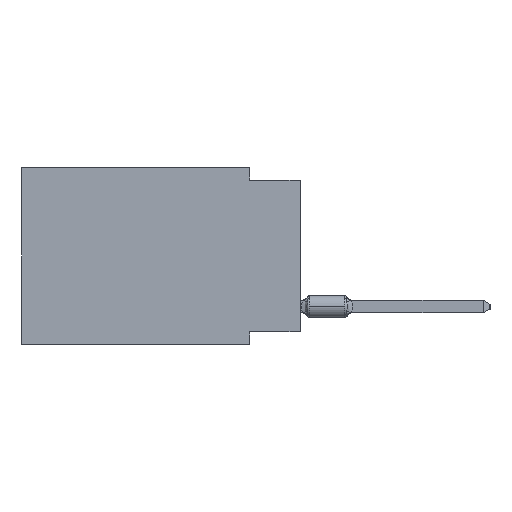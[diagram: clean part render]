
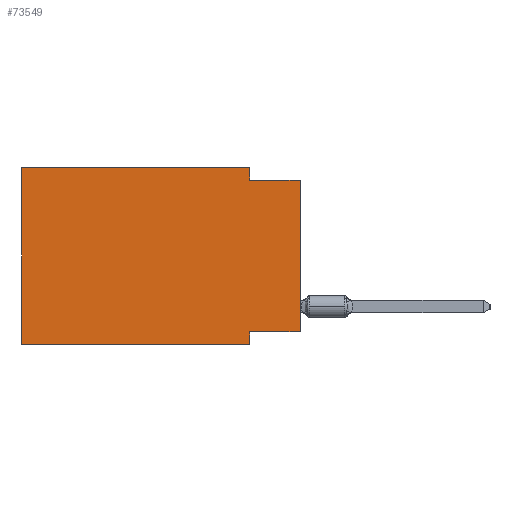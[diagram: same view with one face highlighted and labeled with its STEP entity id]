
A CAD part, left-side view. The second image highlights one B-rep face of the part: STEP entity #73549.
In plain terms, the highlighted planar face has unit normal (-1, 0, 0).
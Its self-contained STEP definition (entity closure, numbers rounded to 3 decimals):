
#684 = VERTEX_POINT ( 'NONE', #69569 ) ;
#3861 = LINE ( 'NONE', #26258, #43445 ) ;
#5385 = CARTESIAN_POINT ( 'NONE',  ( 0., 2.54, -8.89 ) ) ;
#7971 = CARTESIAN_POINT ( 'NONE',  ( 0., 0., -0.635 ) ) ;
#9413 = ORIENTED_EDGE ( 'NONE', *, *, #15101, .T. ) ;
#12250 = ORIENTED_EDGE ( 'NONE', *, *, #73054, .F. ) ;
#12953 = CARTESIAN_POINT ( 'NONE',  ( 0., 2.54, -8.255 ) ) ;
#13824 = VECTOR ( 'NONE', #46925, 1000. ) ;
#14258 = VECTOR ( 'NONE', #72425, 1000. ) ;
#15101 = EDGE_CURVE ( 'NONE', #84694, #73903, #57664, .T. ) ;
#19069 = ORIENTED_EDGE ( 'NONE', *, *, #36887, .F. ) ;
#21084 = LINE ( 'NONE', #55580, #50483 ) ;
#23249 = LINE ( 'NONE', #50221, #69173 ) ;
#25479 = ORIENTED_EDGE ( 'NONE', *, *, #57458, .F. ) ;
#26258 = CARTESIAN_POINT ( 'NONE',  ( 0., 0., 0. ) ) ;
#26704 = ORIENTED_EDGE ( 'NONE', *, *, #41740, .F. ) ;
#27658 = EDGE_CURVE ( 'NONE', #56203, #79455, #86277, .T. ) ;
#30993 = CARTESIAN_POINT ( 'NONE',  ( 0., 2.54, -8.89 ) ) ;
#31537 = FACE_OUTER_BOUND ( 'NONE', #66241, .T. ) ;
#31727 = LINE ( 'NONE', #43693, #14258 ) ;
#32801 = CARTESIAN_POINT ( 'NONE',  ( 0., 2.54, 0. ) ) ;
#36490 = VECTOR ( 'NONE', #80050, 1000. ) ;
#36887 = EDGE_CURVE ( 'NONE', #64367, #86631, #31727, .T. ) ;
#39277 = VECTOR ( 'NONE', #86770, 1000. ) ;
#41740 = EDGE_CURVE ( 'NONE', #684, #67649, #53551, .T. ) ;
#41781 = EDGE_CURVE ( 'NONE', #67649, #73903, #52700, .T. ) ;
#43445 = VECTOR ( 'NONE', #64884, 1000. ) ;
#43693 = CARTESIAN_POINT ( 'NONE',  ( 0., 0., -0.635 ) ) ;
#43954 = CARTESIAN_POINT ( 'NONE',  ( 0., 2.54, -0.635 ) ) ;
#46405 = CARTESIAN_POINT ( 'NONE',  ( 0., 13.97, -8.89 ) ) ;
#46925 = DIRECTION ( 'NONE',  ( 0., 0., -1. ) ) ;
#50221 = CARTESIAN_POINT ( 'NONE',  ( 0., 2.54, 0. ) ) ;
#50483 = VECTOR ( 'NONE', #68862, 1000. ) ;
#52297 = AXIS2_PLACEMENT_3D ( 'NONE', #52738, #79736, #72233 ) ;
#52700 = LINE ( 'NONE', #5385, #13824 ) ;
#52738 = CARTESIAN_POINT ( 'NONE',  ( 0., 13.97, 0. ) ) ;
#53551 = LINE ( 'NONE', #60193, #39277 ) ;
#55580 = CARTESIAN_POINT ( 'NONE',  ( 0., 13.97, 0. ) ) ;
#56203 = VERTEX_POINT ( 'NONE', #60008 ) ;
#56802 = DIRECTION ( 'NONE',  ( 0., -1., 0. ) ) ;
#57228 = CARTESIAN_POINT ( 'NONE',  ( 0., 13.97, -8.89 ) ) ;
#57458 = EDGE_CURVE ( 'NONE', #84694, #56203, #21084, .T. ) ;
#57664 = LINE ( 'NONE', #57228, #66122 ) ;
#59906 = DIRECTION ( 'NONE',  ( 0., 0., -1. ) ) ;
#60008 = CARTESIAN_POINT ( 'NONE',  ( 0., 13.97, 0. ) ) ;
#60193 = CARTESIAN_POINT ( 'NONE',  ( 0., 0., -8.255 ) ) ;
#64367 = VERTEX_POINT ( 'NONE', #43954 ) ;
#64884 = DIRECTION ( 'NONE',  ( 0., 0., 1. ) ) ;
#66122 = VECTOR ( 'NONE', #56802, 1000. ) ;
#66241 = EDGE_LOOP ( 'NONE', ( #79836, #19069, #12250, #69041, #25479, #9413, #79069, #26704 ) ) ;
#66777 = CARTESIAN_POINT ( 'NONE',  ( 0., 13.97, 0. ) ) ;
#67649 = VERTEX_POINT ( 'NONE', #12953 ) ;
#68862 = DIRECTION ( 'NONE',  ( 0., 0., 1. ) ) ;
#69041 = ORIENTED_EDGE ( 'NONE', *, *, #27658, .F. ) ;
#69173 = VECTOR ( 'NONE', #59906, 1000. ) ;
#69569 = CARTESIAN_POINT ( 'NONE',  ( 0., 0., -8.255 ) ) ;
#71784 = PLANE ( 'NONE',  #52297 ) ;
#72233 = DIRECTION ( 'NONE',  ( 0., 0., -1. ) ) ;
#72425 = DIRECTION ( 'NONE',  ( 0., -1., 0. ) ) ;
#73054 = EDGE_CURVE ( 'NONE', #79455, #64367, #23249, .T. ) ;
#73549 = ADVANCED_FACE ( 'NONE', ( #31537 ), #71784, .F. ) ;
#73903 = VERTEX_POINT ( 'NONE', #30993 ) ;
#79069 = ORIENTED_EDGE ( 'NONE', *, *, #41781, .F. ) ;
#79455 = VERTEX_POINT ( 'NONE', #32801 ) ;
#79736 = DIRECTION ( 'NONE',  ( 1., 0., 0. ) ) ;
#79836 = ORIENTED_EDGE ( 'NONE', *, *, #82665, .T. ) ;
#80050 = DIRECTION ( 'NONE',  ( 0., -1., 0. ) ) ;
#82665 = EDGE_CURVE ( 'NONE', #684, #86631, #3861, .T. ) ;
#84694 = VERTEX_POINT ( 'NONE', #46405 ) ;
#86277 = LINE ( 'NONE', #66777, #36490 ) ;
#86631 = VERTEX_POINT ( 'NONE', #7971 ) ;
#86770 = DIRECTION ( 'NONE',  ( 0., 1., 0. ) ) ;
